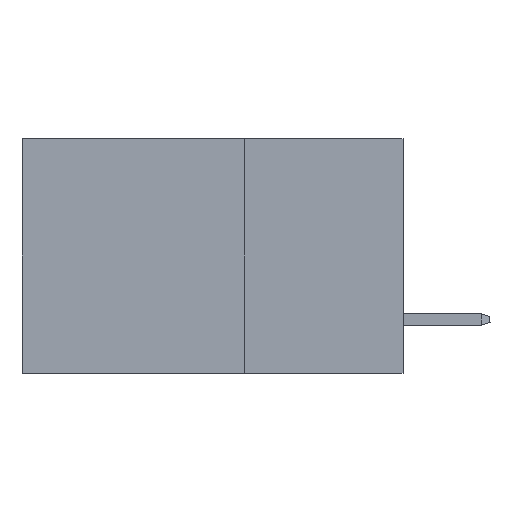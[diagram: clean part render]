
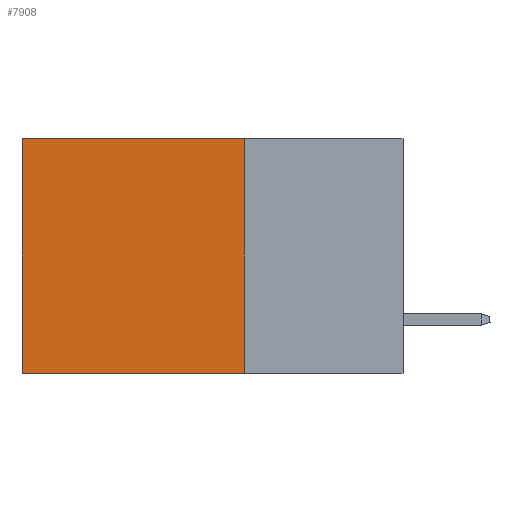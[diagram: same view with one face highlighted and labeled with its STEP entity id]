
A CAD part, left-side view. The second image highlights one B-rep face of the part: STEP entity #7908.
In plain terms, the highlighted planar face has unit normal (-1, 0, 0).
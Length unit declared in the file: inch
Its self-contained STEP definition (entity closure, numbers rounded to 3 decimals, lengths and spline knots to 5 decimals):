
#685 = FACE_OUTER_BOUND ( 'NONE', #25996, .T. ) ;
#1803 = AXIS2_PLACEMENT_3D ( 'NONE', #9125, #13408, #21840 ) ;
#2652 = EDGE_CURVE ( 'NONE', #24010, #21523, #8771, .T. ) ;
#3098 = EDGE_CURVE ( 'NONE', #20862, #24010, #4451, .T. ) ;
#4296 = LINE ( 'NONE', #10245, #21412 ) ;
#4451 = LINE ( 'NONE', #13158, #25679 ) ;
#4976 = PLANE ( 'NONE',  #1803 ) ;
#5679 = ORIENTED_EDGE ( 'NONE', *, *, #22639, .T. ) ;
#5909 = VECTOR ( 'NONE', #25847, 39.37008 ) ;
#7908 = ADVANCED_FACE ( 'NONE', ( #685 ), #4976, .F. ) ;
#8771 = LINE ( 'NONE', #17195, #14603 ) ;
#9125 = CARTESIAN_POINT ( 'NONE',  ( 0.2875, 0.25, 0. ) ) ;
#10245 = CARTESIAN_POINT ( 'NONE',  ( 0.2875, 0.6, 0. ) ) ;
#11178 = CARTESIAN_POINT ( 'NONE',  ( 0.2875, 0.25, 0. ) ) ;
#11913 = ORIENTED_EDGE ( 'NONE', *, *, #13637, .T. ) ;
#12289 = ORIENTED_EDGE ( 'NONE', *, *, #3098, .F. ) ;
#13158 = CARTESIAN_POINT ( 'NONE',  ( 0.2875, 0.25, 0. ) ) ;
#13408 = DIRECTION ( 'NONE',  ( 1., 0., 0. ) ) ;
#13637 = EDGE_CURVE ( 'NONE', #16489, #21523, #4296, .T. ) ;
#14603 = VECTOR ( 'NONE', #15273, 39.37008 ) ;
#15273 = DIRECTION ( 'NONE',  ( 0., 1., 0. ) ) ;
#16489 = VERTEX_POINT ( 'NONE', #16920 ) ;
#16920 = CARTESIAN_POINT ( 'NONE',  ( 0.2875, 0.6, 0. ) ) ;
#17195 = CARTESIAN_POINT ( 'NONE',  ( 0.2875, 0.25, -0.37 ) ) ;
#18549 = DIRECTION ( 'NONE',  ( 0., 0., -1. ) ) ;
#20675 = CARTESIAN_POINT ( 'NONE',  ( 0.2875, 0.6, -0.37 ) ) ;
#20862 = VERTEX_POINT ( 'NONE', #25878 ) ;
#21172 = DIRECTION ( 'NONE',  ( 0., 0., -1. ) ) ;
#21412 = VECTOR ( 'NONE', #18549, 39.37008 ) ;
#21523 = VERTEX_POINT ( 'NONE', #20675 ) ;
#21753 = CARTESIAN_POINT ( 'NONE',  ( 0.2875, 0.25, -0.37 ) ) ;
#21840 = DIRECTION ( 'NONE',  ( 0., 0., -1. ) ) ;
#22639 = EDGE_CURVE ( 'NONE', #20862, #16489, #23782, .T. ) ;
#23782 = LINE ( 'NONE', #11178, #5909 ) ;
#24010 = VERTEX_POINT ( 'NONE', #21753 ) ;
#25679 = VECTOR ( 'NONE', #21172, 39.37008 ) ;
#25847 = DIRECTION ( 'NONE',  ( 0., 1., 0. ) ) ;
#25878 = CARTESIAN_POINT ( 'NONE',  ( 0.2875, 0.25, 0. ) ) ;
#25996 = EDGE_LOOP ( 'NONE', ( #11913, #26095, #12289, #5679 ) ) ;
#26095 = ORIENTED_EDGE ( 'NONE', *, *, #2652, .F. ) ;
